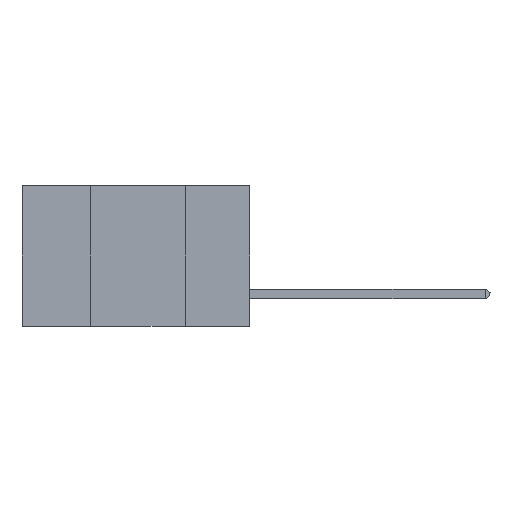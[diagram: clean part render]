
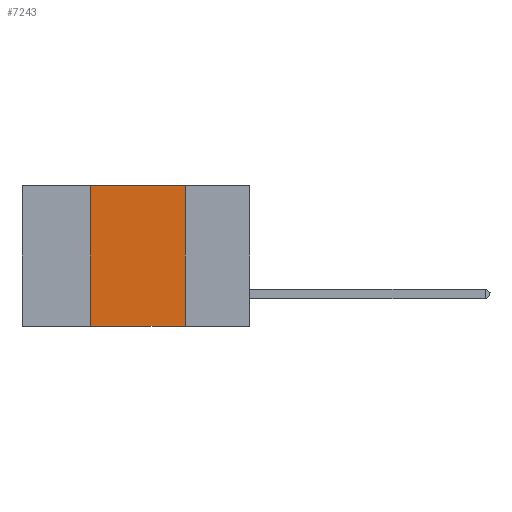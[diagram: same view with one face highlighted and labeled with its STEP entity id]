
A CAD part, left-side view. The second image highlights one B-rep face of the part: STEP entity #7243.
In plain terms, the highlighted planar face has unit normal (-1, 0, 0).
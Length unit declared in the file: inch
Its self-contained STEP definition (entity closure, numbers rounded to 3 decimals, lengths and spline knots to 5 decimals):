
#309 = AXIS2_PLACEMENT_3D ( 'NONE', #4518, #2157, #3311 ) ;
#553 = ORIENTED_EDGE ( 'NONE', *, *, #5531, .F. ) ;
#1332 = DIRECTION ( 'NONE',  ( 0., 0., 1. ) ) ;
#2157 = DIRECTION ( 'NONE',  ( 1., 0., 0. ) ) ;
#2174 = ORIENTED_EDGE ( 'NONE', *, *, #3001, .F. ) ;
#2637 = VERTEX_POINT ( 'NONE', #2720 ) ;
#2720 = CARTESIAN_POINT ( 'NONE',  ( 0., 0.17, 0. ) ) ;
#3001 = EDGE_CURVE ( 'NONE', #8581, #5898, #4257, .T. ) ;
#3311 = DIRECTION ( 'NONE',  ( 0., 0., -1. ) ) ;
#4257 = LINE ( 'NONE', #4825, #11756 ) ;
#4518 = CARTESIAN_POINT ( 'NONE',  ( 0., 0.6, 0. ) ) ;
#4825 = CARTESIAN_POINT ( 'NONE',  ( 0., 0.42, 0. ) ) ;
#4978 = CARTESIAN_POINT ( 'NONE',  ( 0., 0.6, 0. ) ) ;
#5125 = LINE ( 'NONE', #8976, #14197 ) ;
#5531 = EDGE_CURVE ( 'NONE', #2637, #8258, #9722, .T. ) ;
#5898 = VERTEX_POINT ( 'NONE', #6554 ) ;
#6554 = CARTESIAN_POINT ( 'NONE',  ( 0., 0.42, 0. ) ) ;
#7243 = ADVANCED_FACE ( 'NONE', ( #10417 ), #9025, .F. ) ;
#8163 = VECTOR ( 'NONE', #8418, 39.37008 ) ;
#8175 = DIRECTION ( 'NONE',  ( 0., 0., -1. ) ) ;
#8258 = VERTEX_POINT ( 'NONE', #8814 ) ;
#8418 = DIRECTION ( 'NONE',  ( 0., -1., 0. ) ) ;
#8581 = VERTEX_POINT ( 'NONE', #14083 ) ;
#8593 = EDGE_LOOP ( 'NONE', ( #553, #12372, #2174, #9379 ) ) ;
#8604 = EDGE_CURVE ( 'NONE', #8581, #8258, #5125, .T. ) ;
#8814 = CARTESIAN_POINT ( 'NONE',  ( 0., 0.17, -0.37 ) ) ;
#8976 = CARTESIAN_POINT ( 'NONE',  ( 0., 0.6, -0.37 ) ) ;
#9025 = PLANE ( 'NONE',  #309 ) ;
#9137 = CARTESIAN_POINT ( 'NONE',  ( 0., 0.17, 0. ) ) ;
#9379 = ORIENTED_EDGE ( 'NONE', *, *, #8604, .T. ) ;
#9722 = LINE ( 'NONE', #9137, #11088 ) ;
#10417 = FACE_OUTER_BOUND ( 'NONE', #8593, .T. ) ;
#11088 = VECTOR ( 'NONE', #8175, 39.37008 ) ;
#11247 = LINE ( 'NONE', #4978, #8163 ) ;
#11756 = VECTOR ( 'NONE', #1332, 39.37008 ) ;
#12121 = DIRECTION ( 'NONE',  ( 0., -1., 0. ) ) ;
#12372 = ORIENTED_EDGE ( 'NONE', *, *, #14424, .F. ) ;
#14083 = CARTESIAN_POINT ( 'NONE',  ( 0., 0.42, -0.37 ) ) ;
#14197 = VECTOR ( 'NONE', #12121, 39.37008 ) ;
#14424 = EDGE_CURVE ( 'NONE', #5898, #2637, #11247, .T. ) ;
